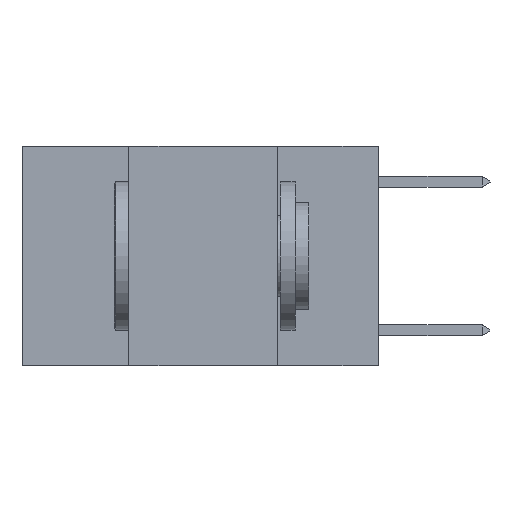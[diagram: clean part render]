
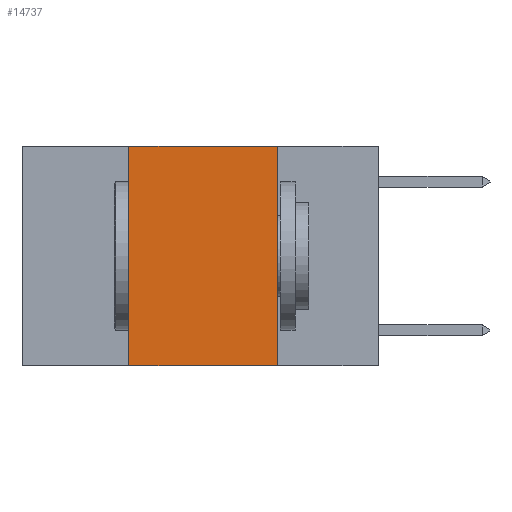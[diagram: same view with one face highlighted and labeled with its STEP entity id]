
A CAD part, left-side view. The second image highlights one B-rep face of the part: STEP entity #14737.
In plain terms, the highlighted planar face has unit normal (-1, 0, 0).
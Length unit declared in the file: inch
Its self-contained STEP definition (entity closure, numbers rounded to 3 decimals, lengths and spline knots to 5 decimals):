
#484 = VECTOR ( 'NONE', #6708, 39.37008 ) ;
#614 = EDGE_CURVE ( 'NONE', #11804, #8933, #12688, .T. ) ;
#1319 = CARTESIAN_POINT ( 'NONE',  ( 0., 0.6, 0. ) ) ;
#1799 = CARTESIAN_POINT ( 'NONE',  ( 0., 0.17, 0. ) ) ;
#3624 = ORIENTED_EDGE ( 'NONE', *, *, #14532, .F. ) ;
#3658 = LINE ( 'NONE', #1799, #15032 ) ;
#4734 = VECTOR ( 'NONE', #20790, 39.37008 ) ;
#5708 = CARTESIAN_POINT ( 'NONE',  ( 0., 0.17, -0.37 ) ) ;
#6013 = CARTESIAN_POINT ( 'NONE',  ( 0., 0.6, 0. ) ) ;
#6576 = DIRECTION ( 'NONE',  ( 0., 0., -1. ) ) ;
#6667 = LINE ( 'NONE', #13280, #13069 ) ;
#6708 = DIRECTION ( 'NONE',  ( 0., -1., 0. ) ) ;
#7436 = ORIENTED_EDGE ( 'NONE', *, *, #10379, .F. ) ;
#7848 = VERTEX_POINT ( 'NONE', #14702 ) ;
#8933 = VERTEX_POINT ( 'NONE', #5708 ) ;
#10080 = CARTESIAN_POINT ( 'NONE',  ( 0., 0.42, -0.37 ) ) ;
#10379 = EDGE_CURVE ( 'NONE', #15919, #8933, #3658, .T. ) ;
#10678 = ORIENTED_EDGE ( 'NONE', *, *, #614, .T. ) ;
#11804 = VERTEX_POINT ( 'NONE', #10080 ) ;
#12688 = LINE ( 'NONE', #19297, #484 ) ;
#13069 = VECTOR ( 'NONE', #19793, 39.37008 ) ;
#13280 = CARTESIAN_POINT ( 'NONE',  ( 0., 0.42, 0. ) ) ;
#13457 = DIRECTION ( 'NONE',  ( 0., 0., -1. ) ) ;
#14532 = EDGE_CURVE ( 'NONE', #11804, #7848, #6667, .T. ) ;
#14702 = CARTESIAN_POINT ( 'NONE',  ( 0., 0.42, 0. ) ) ;
#14737 = ADVANCED_FACE ( 'NONE', ( #15047 ), #19704, .F. ) ;
#15032 = VECTOR ( 'NONE', #13457, 39.37008 ) ;
#15047 = FACE_OUTER_BOUND ( 'NONE', #19412, .T. ) ;
#15919 = VERTEX_POINT ( 'NONE', #18078 ) ;
#16242 = EDGE_CURVE ( 'NONE', #7848, #15919, #19027, .T. ) ;
#16646 = DIRECTION ( 'NONE',  ( 1., 0., 0. ) ) ;
#18078 = CARTESIAN_POINT ( 'NONE',  ( 0., 0.17, 0. ) ) ;
#19027 = LINE ( 'NONE', #6013, #4734 ) ;
#19297 = CARTESIAN_POINT ( 'NONE',  ( 0., 0.6, -0.37 ) ) ;
#19412 = EDGE_LOOP ( 'NONE', ( #7436, #19797, #3624, #10678 ) ) ;
#19661 = AXIS2_PLACEMENT_3D ( 'NONE', #1319, #16646, #6576 ) ;
#19704 = PLANE ( 'NONE',  #19661 ) ;
#19793 = DIRECTION ( 'NONE',  ( 0., 0., 1. ) ) ;
#19797 = ORIENTED_EDGE ( 'NONE', *, *, #16242, .F. ) ;
#20790 = DIRECTION ( 'NONE',  ( 0., -1., 0. ) ) ;
